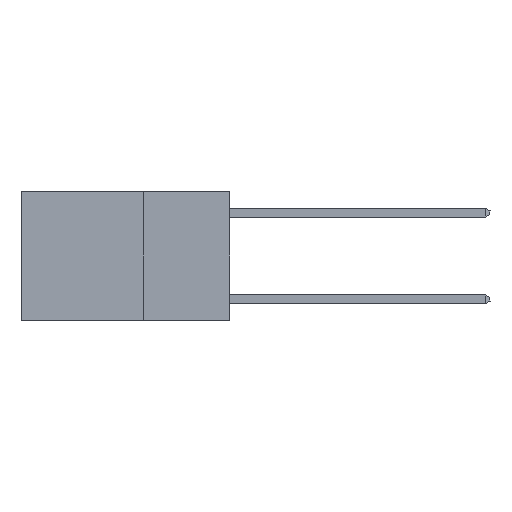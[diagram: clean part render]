
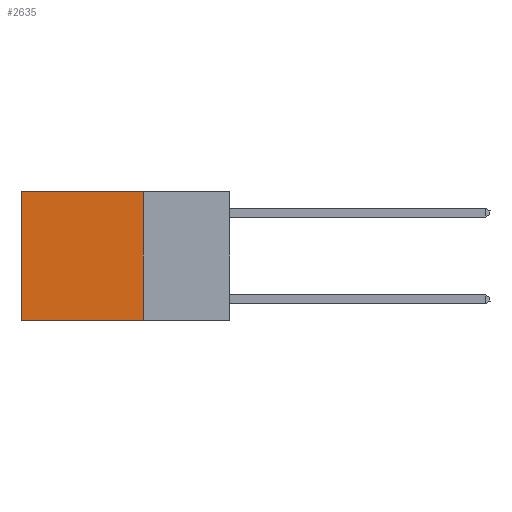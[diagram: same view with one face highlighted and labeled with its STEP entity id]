
A CAD part, left-side view. The second image highlights one B-rep face of the part: STEP entity #2635.
In plain terms, the highlighted planar face has unit normal (-1, 0, 0).
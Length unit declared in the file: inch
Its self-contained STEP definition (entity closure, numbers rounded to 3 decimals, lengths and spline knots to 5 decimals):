
#463 = VERTEX_POINT ( 'NONE', #3370 ) ;
#495 = CARTESIAN_POINT ( 'NONE',  ( 0.2625, 0.6, 0. ) ) ;
#982 = DIRECTION ( 'NONE',  ( 0., 0., -1. ) ) ;
#1166 = EDGE_LOOP ( 'NONE', ( #10721, #15794, #21032, #10453 ) ) ;
#2005 = EDGE_CURVE ( 'NONE', #7538, #17792, #10088, .T. ) ;
#2635 = ADVANCED_FACE ( 'NONE', ( #9194 ), #5617, .F. ) ;
#3370 = CARTESIAN_POINT ( 'NONE',  ( 0.2625, 0.6, -0.37 ) ) ;
#3887 = VECTOR ( 'NONE', #5559, 39.37008 ) ;
#4005 = CARTESIAN_POINT ( 'NONE',  ( 0.2625, 0.25, 0. ) ) ;
#4083 = CARTESIAN_POINT ( 'NONE',  ( 0.2625, 0.25, 0. ) ) ;
#4090 = CARTESIAN_POINT ( 'NONE',  ( 0.2625, 0.25, 0. ) ) ;
#4847 = VECTOR ( 'NONE', #7174, 39.37008 ) ;
#4914 = CARTESIAN_POINT ( 'NONE',  ( 0.2625, 0.6, 0. ) ) ;
#5559 = DIRECTION ( 'NONE',  ( 0., 1., 0. ) ) ;
#5617 = PLANE ( 'NONE',  #10770 ) ;
#6256 = VECTOR ( 'NONE', #16399, 39.37008 ) ;
#7174 = DIRECTION ( 'NONE',  ( 0., 1., 0. ) ) ;
#7376 = EDGE_CURVE ( 'NONE', #7538, #11453, #18576, .T. ) ;
#7538 = VERTEX_POINT ( 'NONE', #4090 ) ;
#7646 = VECTOR ( 'NONE', #9682, 39.37008 ) ;
#9194 = FACE_OUTER_BOUND ( 'NONE', #1166, .T. ) ;
#9682 = DIRECTION ( 'NONE',  ( 0., 0., -1. ) ) ;
#10088 = LINE ( 'NONE', #10515, #6256 ) ;
#10220 = CARTESIAN_POINT ( 'NONE',  ( 0.2625, 0.25, -0.37 ) ) ;
#10453 = ORIENTED_EDGE ( 'NONE', *, *, #7376, .T. ) ;
#10515 = CARTESIAN_POINT ( 'NONE',  ( 0.2625, 0.25, 0. ) ) ;
#10721 = ORIENTED_EDGE ( 'NONE', *, *, #19369, .T. ) ;
#10770 = AXIS2_PLACEMENT_3D ( 'NONE', #4083, #16133, #982 ) ;
#11453 = VERTEX_POINT ( 'NONE', #495 ) ;
#15794 = ORIENTED_EDGE ( 'NONE', *, *, #16297, .F. ) ;
#16133 = DIRECTION ( 'NONE',  ( 1., 0., 0. ) ) ;
#16297 = EDGE_CURVE ( 'NONE', #17792, #463, #20464, .T. ) ;
#16399 = DIRECTION ( 'NONE',  ( 0., 0., -1. ) ) ;
#17792 = VERTEX_POINT ( 'NONE', #20982 ) ;
#18576 = LINE ( 'NONE', #4005, #4847 ) ;
#19369 = EDGE_CURVE ( 'NONE', #11453, #463, #21548, .T. ) ;
#20464 = LINE ( 'NONE', #10220, #3887 ) ;
#20982 = CARTESIAN_POINT ( 'NONE',  ( 0.2625, 0.25, -0.37 ) ) ;
#21032 = ORIENTED_EDGE ( 'NONE', *, *, #2005, .F. ) ;
#21548 = LINE ( 'NONE', #4914, #7646 ) ;
